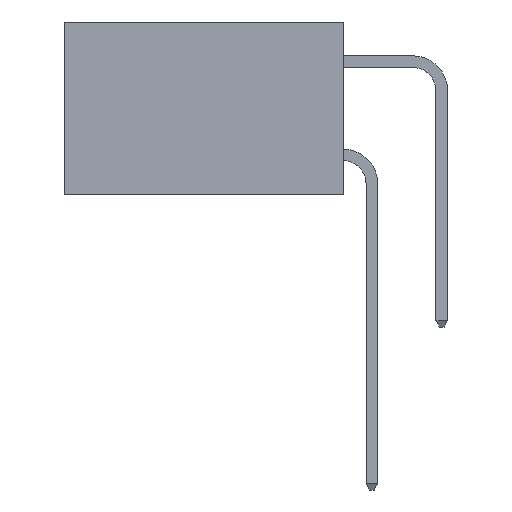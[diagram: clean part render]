
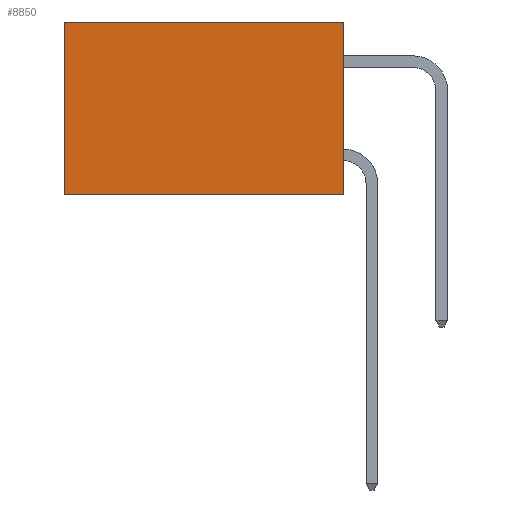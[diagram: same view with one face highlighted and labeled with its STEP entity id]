
A CAD part, left-side view. The second image highlights one B-rep face of the part: STEP entity #8850.
In plain terms, the highlighted planar face has unit normal (-1, 0, 0).
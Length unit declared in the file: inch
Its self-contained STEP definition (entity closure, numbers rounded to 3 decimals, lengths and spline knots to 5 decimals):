
#2660 = VERTEX_POINT ( 'NONE', #7283 ) ;
#2720 = CARTESIAN_POINT ( 'NONE',  ( 0.2615, 0., -0.37 ) ) ;
#4172 = LINE ( 'NONE', #11271, #20563 ) ;
#4665 = FACE_OUTER_BOUND ( 'NONE', #24817, .T. ) ;
#5334 = ORIENTED_EDGE ( 'NONE', *, *, #17635, .F. ) ;
#5414 = DIRECTION ( 'NONE',  ( 0., 0., -1. ) ) ;
#7283 = CARTESIAN_POINT ( 'NONE',  ( 0.2615, 0., -0.37 ) ) ;
#7768 = CARTESIAN_POINT ( 'NONE',  ( 0.2615, 0., 0. ) ) ;
#8089 = AXIS2_PLACEMENT_3D ( 'NONE', #22888, #27106, #14470 ) ;
#8727 = VECTOR ( 'NONE', #17789, 39.37008 ) ;
#8850 = ADVANCED_FACE ( 'NONE', ( #4665 ), #25027, .F. ) ;
#10248 = VERTEX_POINT ( 'NONE', #16922 ) ;
#11271 = CARTESIAN_POINT ( 'NONE',  ( 0.2615, 0., -0.37 ) ) ;
#12080 = EDGE_CURVE ( 'NONE', #19028, #2660, #20046, .T. ) ;
#12901 = VERTEX_POINT ( 'NONE', #16163 ) ;
#13264 = VECTOR ( 'NONE', #5414, 39.37008 ) ;
#13936 = LINE ( 'NONE', #18109, #13264 ) ;
#14470 = DIRECTION ( 'NONE',  ( 0., 0., -1. ) ) ;
#14869 = EDGE_CURVE ( 'NONE', #10248, #12901, #13936, .T. ) ;
#15194 = EDGE_CURVE ( 'NONE', #19028, #10248, #22226, .T. ) ;
#15524 = ORIENTED_EDGE ( 'NONE', *, *, #14869, .T. ) ;
#16163 = CARTESIAN_POINT ( 'NONE',  ( 0.2615, 0.6, -0.37 ) ) ;
#16922 = CARTESIAN_POINT ( 'NONE',  ( 0.2615, 0.6, 0. ) ) ;
#17546 = ORIENTED_EDGE ( 'NONE', *, *, #15194, .T. ) ;
#17635 = EDGE_CURVE ( 'NONE', #2660, #12901, #4172, .T. ) ;
#17789 = DIRECTION ( 'NONE',  ( 0., 0., -1. ) ) ;
#18109 = CARTESIAN_POINT ( 'NONE',  ( 0.2615, 0.6, -0.37 ) ) ;
#19028 = VERTEX_POINT ( 'NONE', #23369 ) ;
#19723 = ORIENTED_EDGE ( 'NONE', *, *, #12080, .F. ) ;
#20046 = LINE ( 'NONE', #2720, #8727 ) ;
#20563 = VECTOR ( 'NONE', #24011, 39.37008 ) ;
#22226 = LINE ( 'NONE', #7768, #27136 ) ;
#22888 = CARTESIAN_POINT ( 'NONE',  ( 0.2615, 0., -0.37 ) ) ;
#23369 = CARTESIAN_POINT ( 'NONE',  ( 0.2615, 0., 0. ) ) ;
#24011 = DIRECTION ( 'NONE',  ( 0., 1., 0. ) ) ;
#24754 = DIRECTION ( 'NONE',  ( 0., 1., 0. ) ) ;
#24817 = EDGE_LOOP ( 'NONE', ( #15524, #5334, #19723, #17546 ) ) ;
#25027 = PLANE ( 'NONE',  #8089 ) ;
#27106 = DIRECTION ( 'NONE',  ( 1., 0., 0. ) ) ;
#27136 = VECTOR ( 'NONE', #24754, 39.37008 ) ;
